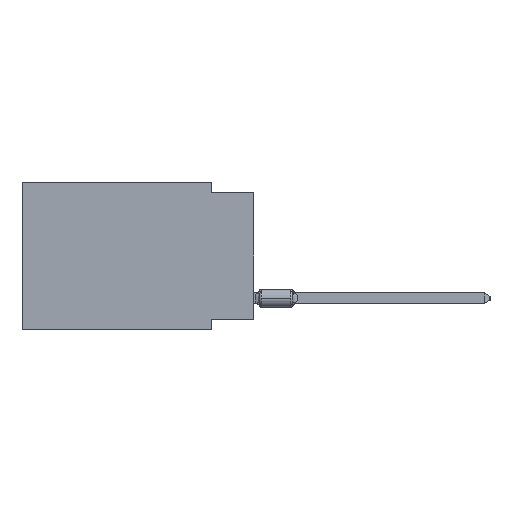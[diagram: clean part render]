
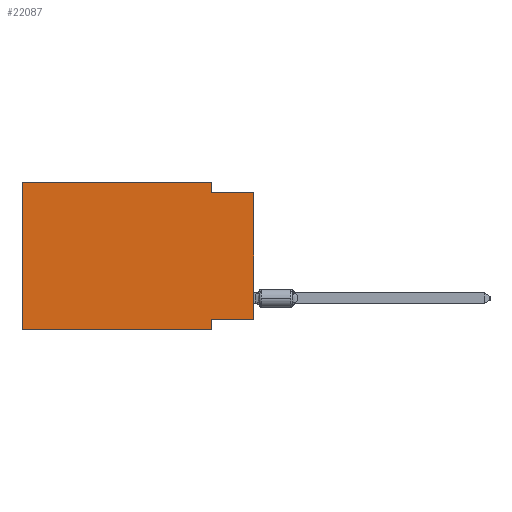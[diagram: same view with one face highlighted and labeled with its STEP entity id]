
A CAD part, left-side view. The second image highlights one B-rep face of the part: STEP entity #22087.
In plain terms, the highlighted planar face has unit normal (-1, 0, 0).
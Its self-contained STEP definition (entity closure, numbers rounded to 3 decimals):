
#480 = DIRECTION ( 'NONE',  ( 0., -1., 0. ) ) ;
#659 = EDGE_CURVE ( 'NONE', #33559, #16148, #18618, .T. ) ;
#728 = EDGE_CURVE ( 'NONE', #29412, #31419, #10934, .T. ) ;
#967 = CARTESIAN_POINT ( 'NONE',  ( 0., 2.54, 0. ) ) ;
#1775 = DIRECTION ( 'NONE',  ( 1., 0., 0. ) ) ;
#2678 = VECTOR ( 'NONE', #7819, 1000. ) ;
#4330 = CARTESIAN_POINT ( 'NONE',  ( 0., 2.54, -0.635 ) ) ;
#4674 = LINE ( 'NONE', #5340, #29745 ) ;
#5194 = CARTESIAN_POINT ( 'NONE',  ( 0., 13.97, 0. ) ) ;
#5340 = CARTESIAN_POINT ( 'NONE',  ( 0., 13.97, -8.89 ) ) ;
#6192 = VERTEX_POINT ( 'NONE', #8619 ) ;
#7325 = CARTESIAN_POINT ( 'NONE',  ( 0., 0., 0. ) ) ;
#7371 = CARTESIAN_POINT ( 'NONE',  ( 0., 13.97, 0. ) ) ;
#7647 = DIRECTION ( 'NONE',  ( 0., -1., 0. ) ) ;
#7819 = DIRECTION ( 'NONE',  ( 0., 0., 1. ) ) ;
#8316 = EDGE_LOOP ( 'NONE', ( #9476, #19492, #15905, #23196, #14161, #25647, #9002, #20788 ) ) ;
#8344 = CARTESIAN_POINT ( 'NONE',  ( 0., 0., -0.635 ) ) ;
#8619 = CARTESIAN_POINT ( 'NONE',  ( 0., 0., -0.635 ) ) ;
#9002 = ORIENTED_EDGE ( 'NONE', *, *, #23546, .F. ) ;
#9476 = ORIENTED_EDGE ( 'NONE', *, *, #12764, .T. ) ;
#9592 = DIRECTION ( 'NONE',  ( 0., 0., 1. ) ) ;
#9636 = DIRECTION ( 'NONE',  ( 0., 0., -1. ) ) ;
#10934 = LINE ( 'NONE', #19306, #30807 ) ;
#11181 = DIRECTION ( 'NONE',  ( 0., 0., -1. ) ) ;
#11257 = VECTOR ( 'NONE', #9592, 1000. ) ;
#12588 = PLANE ( 'NONE',  #34194 ) ;
#12764 = EDGE_CURVE ( 'NONE', #29412, #6192, #25461, .T. ) ;
#14161 = ORIENTED_EDGE ( 'NONE', *, *, #30394, .F. ) ;
#14649 = VECTOR ( 'NONE', #7647, 1000. ) ;
#15663 = LINE ( 'NONE', #28757, #2678 ) ;
#15905 = ORIENTED_EDGE ( 'NONE', *, *, #31469, .F. ) ;
#16148 = VERTEX_POINT ( 'NONE', #967 ) ;
#16586 = CARTESIAN_POINT ( 'NONE',  ( 0., 2.54, -8.89 ) ) ;
#17926 = DIRECTION ( 'NONE',  ( 0., -1., 0. ) ) ;
#18618 = LINE ( 'NONE', #5194, #14649 ) ;
#19166 = VECTOR ( 'NONE', #480, 1000. ) ;
#19306 = CARTESIAN_POINT ( 'NONE',  ( 0., 0., -8.255 ) ) ;
#19492 = ORIENTED_EDGE ( 'NONE', *, *, #23887, .F. ) ;
#20788 = ORIENTED_EDGE ( 'NONE', *, *, #728, .F. ) ;
#21741 = DIRECTION ( 'NONE',  ( 0., 1., 0. ) ) ;
#22087 = ADVANCED_FACE ( 'NONE', ( #33854 ), #12588, .F. ) ;
#22179 = DIRECTION ( 'NONE',  ( 0., 0., -1. ) ) ;
#23196 = ORIENTED_EDGE ( 'NONE', *, *, #659, .F. ) ;
#23546 = EDGE_CURVE ( 'NONE', #31419, #24138, #24428, .T. ) ;
#23887 = EDGE_CURVE ( 'NONE', #29162, #6192, #32222, .T. ) ;
#24138 = VERTEX_POINT ( 'NONE', #34295 ) ;
#24158 = EDGE_CURVE ( 'NONE', #33478, #24138, #4674, .T. ) ;
#24428 = LINE ( 'NONE', #16586, #25294 ) ;
#25294 = VECTOR ( 'NONE', #11181, 1000. ) ;
#25461 = LINE ( 'NONE', #7325, #11257 ) ;
#25625 = CARTESIAN_POINT ( 'NONE',  ( 0., 13.97, 0. ) ) ;
#25647 = ORIENTED_EDGE ( 'NONE', *, *, #24158, .T. ) ;
#25805 = CARTESIAN_POINT ( 'NONE',  ( 0., 13.97, -8.89 ) ) ;
#26160 = VECTOR ( 'NONE', #22179, 1000. ) ;
#26568 = CARTESIAN_POINT ( 'NONE',  ( 0., 2.54, -8.255 ) ) ;
#27088 = CARTESIAN_POINT ( 'NONE',  ( 0., 2.54, 0. ) ) ;
#28757 = CARTESIAN_POINT ( 'NONE',  ( 0., 13.97, 0. ) ) ;
#29162 = VERTEX_POINT ( 'NONE', #4330 ) ;
#29412 = VERTEX_POINT ( 'NONE', #33238 ) ;
#29703 = LINE ( 'NONE', #27088, #26160 ) ;
#29745 = VECTOR ( 'NONE', #17926, 1000. ) ;
#30394 = EDGE_CURVE ( 'NONE', #33478, #33559, #15663, .T. ) ;
#30807 = VECTOR ( 'NONE', #21741, 1000. ) ;
#31419 = VERTEX_POINT ( 'NONE', #26568 ) ;
#31469 = EDGE_CURVE ( 'NONE', #16148, #29162, #29703, .T. ) ;
#32222 = LINE ( 'NONE', #8344, #19166 ) ;
#33238 = CARTESIAN_POINT ( 'NONE',  ( 0., 0., -8.255 ) ) ;
#33478 = VERTEX_POINT ( 'NONE', #25805 ) ;
#33559 = VERTEX_POINT ( 'NONE', #25625 ) ;
#33854 = FACE_OUTER_BOUND ( 'NONE', #8316, .T. ) ;
#34194 = AXIS2_PLACEMENT_3D ( 'NONE', #7371, #1775, #9636 ) ;
#34295 = CARTESIAN_POINT ( 'NONE',  ( 0., 2.54, -8.89 ) ) ;
